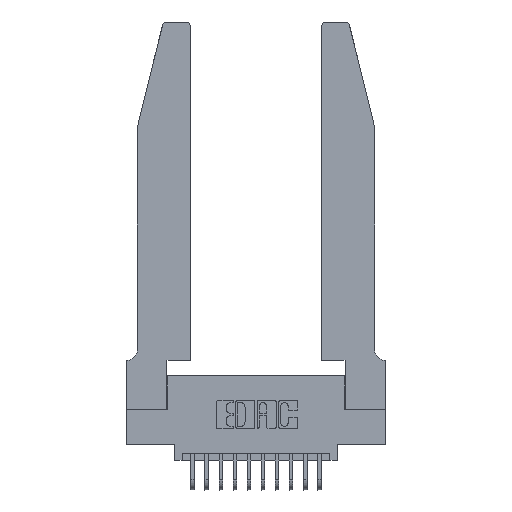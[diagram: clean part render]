
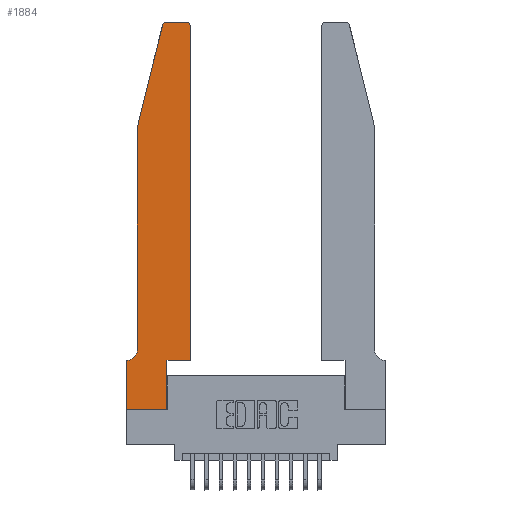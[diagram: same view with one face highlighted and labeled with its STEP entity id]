
A CAD part, top view. The second image highlights one B-rep face of the part: STEP entity #1884.
In plain terms, the highlighted planar face has unit normal (0, 0, 1).
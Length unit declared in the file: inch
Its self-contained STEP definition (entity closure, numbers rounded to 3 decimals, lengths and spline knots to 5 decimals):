
#203 = CARTESIAN_POINT ( 'NONE',  ( 0.0755, 0.42, 0.37 ) ) ;
#502 = VERTEX_POINT ( 'NONE', #2536 ) ;
#542 = VERTEX_POINT ( 'NONE', #7031 ) ;
#555 = VERTEX_POINT ( 'NONE', #13866 ) ;
#790 = CIRCLE ( 'NONE', #16807, 0.03 ) ;
#918 = VERTEX_POINT ( 'NONE', #3209 ) ;
#1047 = ORIENTED_EDGE ( 'NONE', *, *, #6628, .T. ) ;
#1124 = CARTESIAN_POINT ( 'NONE',  ( 0.0755, 0.35, 0.37 ) ) ;
#1194 = DIRECTION ( 'NONE',  ( 0., -1., 0. ) ) ;
#1672 = ORIENTED_EDGE ( 'NONE', *, *, #3186, .T. ) ;
#1884 = ADVANCED_FACE ( 'NONE', ( #7443 ), #12884, .T. ) ;
#1976 = AXIS2_PLACEMENT_3D ( 'NONE', #15128, #6564, #16499 ) ;
#2131 = VERTEX_POINT ( 'NONE', #3997 ) ;
#2536 = CARTESIAN_POINT ( 'NONE',  ( 0.4505, 0.35, 0.37 ) ) ;
#2725 = VECTOR ( 'NONE', #6070, 39.37008 ) ;
#2812 = CARTESIAN_POINT ( 'NONE',  ( 0., 0., 0.37 ) ) ;
#3186 = EDGE_CURVE ( 'NONE', #555, #17086, #11056, .T. ) ;
#3209 = CARTESIAN_POINT ( 'NONE',  ( 0.0755, 2., 0.37 ) ) ;
#3679 = ORIENTED_EDGE ( 'NONE', *, *, #16806, .T. ) ;
#3738 = CARTESIAN_POINT ( 'NONE',  ( 0.2865, 0.35, 0.37 ) ) ;
#3758 = VECTOR ( 'NONE', #13292, 39.37008 ) ;
#3822 = LINE ( 'NONE', #9343, #11560 ) ;
#3997 = CARTESIAN_POINT ( 'NONE',  ( 0.2865, 0.35, 0.37 ) ) ;
#4302 = ORIENTED_EDGE ( 'NONE', *, *, #15147, .T. ) ;
#4613 = CARTESIAN_POINT ( 'NONE',  ( 0., 0., 0.37 ) ) ;
#4641 = ORIENTED_EDGE ( 'NONE', *, *, #17950, .T. ) ;
#4850 = ORIENTED_EDGE ( 'NONE', *, *, #15600, .T. ) ;
#5005 = EDGE_CURVE ( 'NONE', #918, #5708, #10558, .T. ) ;
#5013 = EDGE_CURVE ( 'NONE', #542, #918, #7582, .T. ) ;
#5191 = LINE ( 'NONE', #9294, #12464 ) ;
#5204 = AXIS2_PLACEMENT_3D ( 'NONE', #12943, #16169, #14083 ) ;
#5386 = VERTEX_POINT ( 'NONE', #18039 ) ;
#5489 = DIRECTION ( 'NONE',  ( -1., 0., 0. ) ) ;
#5530 = CIRCLE ( 'NONE', #1976, 0.03 ) ;
#5708 = VERTEX_POINT ( 'NONE', #203 ) ;
#5915 = CARTESIAN_POINT ( 'NONE',  ( 0.4205, 2.72, 0.37 ) ) ;
#6070 = DIRECTION ( 'NONE',  ( 1., 0., 0. ) ) ;
#6564 = DIRECTION ( 'NONE',  ( 0., 0., 1. ) ) ;
#6579 = LINE ( 'NONE', #4613, #2725 ) ;
#6628 = EDGE_CURVE ( 'NONE', #13515, #555, #7746, .T. ) ;
#7002 = DIRECTION ( 'NONE',  ( -1., 0., 0. ) ) ;
#7031 = CARTESIAN_POINT ( 'NONE',  ( 0.25487, 2.72718, 0.37 ) ) ;
#7140 = DIRECTION ( 'NONE',  ( 0., 0., -1. ) ) ;
#7391 = DIRECTION ( 'NONE',  ( 1., 0., 0. ) ) ;
#7415 = CARTESIAN_POINT ( 'NONE',  ( 0.2865, 0., 0.37 ) ) ;
#7443 = FACE_OUTER_BOUND ( 'NONE', #12400, .T. ) ;
#7462 = EDGE_CURVE ( 'NONE', #17086, #17750, #6579, .T. ) ;
#7582 = LINE ( 'NONE', #15666, #17545 ) ;
#7746 = LINE ( 'NONE', #1124, #15329 ) ;
#7950 = ORIENTED_EDGE ( 'NONE', *, *, #5013, .T. ) ;
#8386 = CARTESIAN_POINT ( 'NONE',  ( 0.2605, 2.75, 0.37 ) ) ;
#8392 = ORIENTED_EDGE ( 'NONE', *, *, #5005, .T. ) ;
#9294 = CARTESIAN_POINT ( 'NONE',  ( 0.4505, 0.35, 0.37 ) ) ;
#9343 = CARTESIAN_POINT ( 'NONE',  ( 0.4505, 0.35, 0.37 ) ) ;
#9828 = VECTOR ( 'NONE', #16594, 39.37008 ) ;
#10085 = DIRECTION ( 'NONE',  ( -0.239, -0.971, 0. ) ) ;
#10558 = LINE ( 'NONE', #18467, #15170 ) ;
#10650 = ORIENTED_EDGE ( 'NONE', *, *, #7462, .T. ) ;
#10762 = DIRECTION ( 'NONE',  ( 0., 1., 0. ) ) ;
#10861 = ORIENTED_EDGE ( 'NONE', *, *, #12644, .T. ) ;
#11056 = LINE ( 'NONE', #13235, #3758 ) ;
#11069 = CARTESIAN_POINT ( 'NONE',  ( 0.4205, 2.75, 0.37 ) ) ;
#11293 = AXIS2_PLACEMENT_3D ( 'NONE', #15675, #7140, #17063 ) ;
#11560 = VECTOR ( 'NONE', #17763, 39.37008 ) ;
#12400 = EDGE_LOOP ( 'NONE', ( #10861, #3679, #7950, #8392, #4641, #1047, #1672, #10650, #16230, #15345, #4850, #4302 ) ) ;
#12464 = VECTOR ( 'NONE', #10762, 39.37008 ) ;
#12644 = EDGE_CURVE ( 'NONE', #15752, #5386, #18441, .T. ) ;
#12884 = PLANE ( 'NONE',  #5204 ) ;
#12943 = CARTESIAN_POINT ( 'NONE',  ( 0., 0.35, 0.37 ) ) ;
#13235 = CARTESIAN_POINT ( 'NONE',  ( 0., 0., 0.37 ) ) ;
#13292 = DIRECTION ( 'NONE',  ( 0., -1., 0. ) ) ;
#13515 = VERTEX_POINT ( 'NONE', #16199 ) ;
#13846 = CIRCLE ( 'NONE', #11293, 0.07 ) ;
#13866 = CARTESIAN_POINT ( 'NONE',  ( 0., 0.35, 0.37 ) ) ;
#14083 = DIRECTION ( 'NONE',  ( 1., 0., 0. ) ) ;
#14320 = VECTOR ( 'NONE', #5489, 39.37008 ) ;
#14334 = EDGE_CURVE ( 'NONE', #17750, #2131, #14477, .T. ) ;
#14477 = LINE ( 'NONE', #3738, #9828 ) ;
#15128 = CARTESIAN_POINT ( 'NONE',  ( 0.284, 2.72, 0.37 ) ) ;
#15147 = EDGE_CURVE ( 'NONE', #15444, #15752, #790, .T. ) ;
#15170 = VECTOR ( 'NONE', #1194, 39.37008 ) ;
#15329 = VECTOR ( 'NONE', #7002, 39.37008 ) ;
#15345 = ORIENTED_EDGE ( 'NONE', *, *, #16160, .T. ) ;
#15444 = VERTEX_POINT ( 'NONE', #15947 ) ;
#15600 = EDGE_CURVE ( 'NONE', #502, #15444, #5191, .T. ) ;
#15666 = CARTESIAN_POINT ( 'NONE',  ( 0.0755, 2., 0.37 ) ) ;
#15675 = CARTESIAN_POINT ( 'NONE',  ( 0.0055, 0.42, 0.37 ) ) ;
#15752 = VERTEX_POINT ( 'NONE', #11069 ) ;
#15902 = DIRECTION ( 'NONE',  ( 0., 0., 1. ) ) ;
#15947 = CARTESIAN_POINT ( 'NONE',  ( 0.4505, 2.72, 0.37 ) ) ;
#16160 = EDGE_CURVE ( 'NONE', #2131, #502, #3822, .T. ) ;
#16169 = DIRECTION ( 'NONE',  ( 0., 0., 1. ) ) ;
#16199 = CARTESIAN_POINT ( 'NONE',  ( 0.0055, 0.35, 0.37 ) ) ;
#16230 = ORIENTED_EDGE ( 'NONE', *, *, #14334, .T. ) ;
#16499 = DIRECTION ( 'NONE',  ( 1., 0., 0. ) ) ;
#16594 = DIRECTION ( 'NONE',  ( 0., 1., 0. ) ) ;
#16806 = EDGE_CURVE ( 'NONE', #5386, #542, #5530, .T. ) ;
#16807 = AXIS2_PLACEMENT_3D ( 'NONE', #5915, #15902, #7391 ) ;
#17063 = DIRECTION ( 'NONE',  ( -1., 0., 0. ) ) ;
#17086 = VERTEX_POINT ( 'NONE', #2812 ) ;
#17545 = VECTOR ( 'NONE', #10085, 39.37008 ) ;
#17750 = VERTEX_POINT ( 'NONE', #7415 ) ;
#17763 = DIRECTION ( 'NONE',  ( 1., 0., 0. ) ) ;
#17950 = EDGE_CURVE ( 'NONE', #5708, #13515, #13846, .T. ) ;
#18039 = CARTESIAN_POINT ( 'NONE',  ( 0.284, 2.75, 0.37 ) ) ;
#18441 = LINE ( 'NONE', #8386, #14320 ) ;
#18467 = CARTESIAN_POINT ( 'NONE',  ( 0.0755, 2., 0.37 ) ) ;
